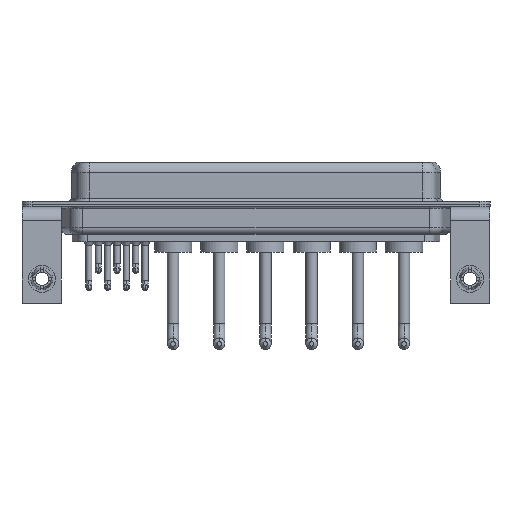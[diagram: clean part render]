
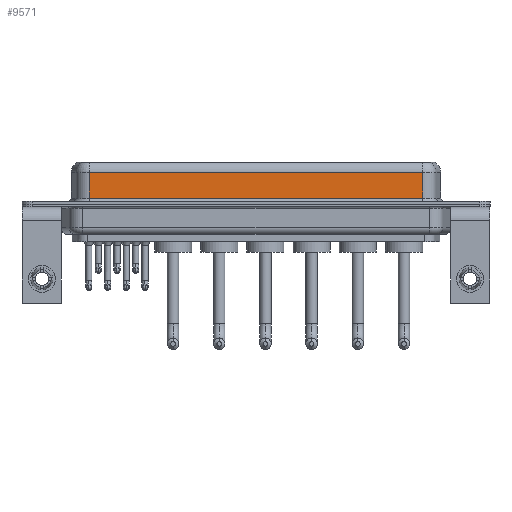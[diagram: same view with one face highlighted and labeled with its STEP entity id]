
A CAD part, front view. The second image highlights one B-rep face of the part: STEP entity #9571.
In plain terms, the highlighted planar face has unit normal (0, -1, 0).
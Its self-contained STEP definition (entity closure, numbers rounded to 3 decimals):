
#364 = ORIENTED_EDGE ( 'NONE', *, *, #17482, .T. ) ;
#674 = DIRECTION ( 'NONE',  ( 0., 0., 1. ) ) ;
#1294 = DIRECTION ( 'NONE',  ( -1., 0., 0. ) ) ;
#1417 = ORIENTED_EDGE ( 'NONE', *, *, #12279, .T. ) ;
#1562 = DIRECTION ( 'NONE',  ( 0., 0., -1. ) ) ;
#2022 = ORIENTED_EDGE ( 'NONE', *, *, #16274, .T. ) ;
#2402 = AXIS2_PLACEMENT_3D ( 'NONE', #13348, #15115, #674 ) ;
#3394 = CARTESIAN_POINT ( 'NONE',  ( 7.038, -3.95, 0.9 ) ) ;
#3520 = LINE ( 'NONE', #9957, #9141 ) ;
#4699 = CARTESIAN_POINT ( 'NONE',  ( 56.462, -3.95, 6.4 ) ) ;
#4801 = LINE ( 'NONE', #4699, #12878 ) ;
#6247 = CARTESIAN_POINT ( 'NONE',  ( 56.462, -3.95, 4.65 ) ) ;
#6567 = DIRECTION ( 'NONE',  ( 0., 0., -1. ) ) ;
#8784 = CARTESIAN_POINT ( 'NONE',  ( 56.462, -3.95, 0.9 ) ) ;
#8901 = LINE ( 'NONE', #8784, #20229 ) ;
#9141 = VECTOR ( 'NONE', #6567, 1000. ) ;
#9527 = VERTEX_POINT ( 'NONE', #11857 ) ;
#9571 = ADVANCED_FACE ( 'NONE', ( #18482 ), #10385, .F. ) ;
#9957 = CARTESIAN_POINT ( 'NONE',  ( 7.038, -3.95, 6.4 ) ) ;
#10385 = PLANE ( 'NONE',  #2402 ) ;
#10485 = EDGE_CURVE ( 'NONE', #20080, #9527, #4801, .T. ) ;
#11104 = LINE ( 'NONE', #6247, #11278 ) ;
#11261 = EDGE_LOOP ( 'NONE', ( #12255, #2022, #1417, #364 ) ) ;
#11278 = VECTOR ( 'NONE', #1294, 1000. ) ;
#11857 = CARTESIAN_POINT ( 'NONE',  ( 56.462, -3.95, 0.9 ) ) ;
#12031 = CARTESIAN_POINT ( 'NONE',  ( 7.038, -3.95, 4.65 ) ) ;
#12255 = ORIENTED_EDGE ( 'NONE', *, *, #10485, .F. ) ;
#12279 = EDGE_CURVE ( 'NONE', #12935, #16487, #3520, .T. ) ;
#12878 = VECTOR ( 'NONE', #1562, 1000. ) ;
#12935 = VERTEX_POINT ( 'NONE', #12031 ) ;
#13348 = CARTESIAN_POINT ( 'NONE',  ( 56.462, -3.95, 6.4 ) ) ;
#13745 = DIRECTION ( 'NONE',  ( 1., 0., 0. ) ) ;
#15115 = DIRECTION ( 'NONE',  ( 0., 1., 0. ) ) ;
#16274 = EDGE_CURVE ( 'NONE', #20080, #12935, #11104, .T. ) ;
#16487 = VERTEX_POINT ( 'NONE', #3394 ) ;
#17482 = EDGE_CURVE ( 'NONE', #16487, #9527, #8901, .T. ) ;
#17621 = CARTESIAN_POINT ( 'NONE',  ( 56.462, -3.95, 4.65 ) ) ;
#18482 = FACE_OUTER_BOUND ( 'NONE', #11261, .T. ) ;
#20080 = VERTEX_POINT ( 'NONE', #17621 ) ;
#20229 = VECTOR ( 'NONE', #13745, 1000. ) ;
